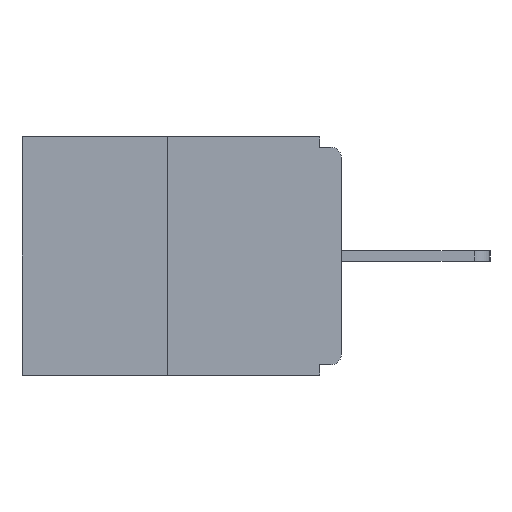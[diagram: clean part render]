
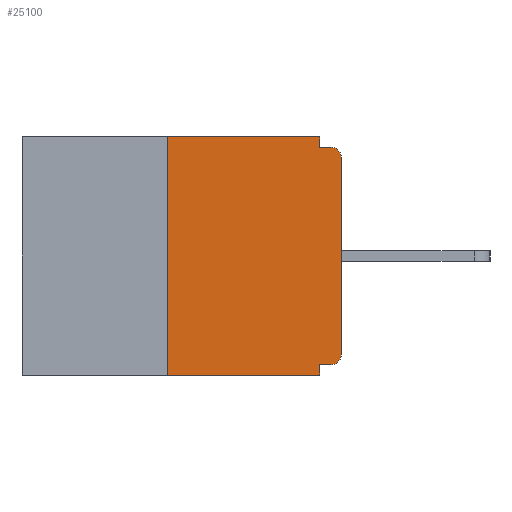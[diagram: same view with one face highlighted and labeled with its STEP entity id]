
A CAD part, left-side view. The second image highlights one B-rep face of the part: STEP entity #25100.
In plain terms, the highlighted planar face has unit normal (-1, 0, 0).
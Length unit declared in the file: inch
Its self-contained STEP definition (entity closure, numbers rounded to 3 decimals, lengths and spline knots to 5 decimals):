
#751 = CARTESIAN_POINT ( 'NONE',  ( 0., 0.031, -0.343 ) ) ;
#800 = CARTESIAN_POINT ( 'NONE',  ( 0., 0.015, -0.015 ) ) ;
#1112 = CARTESIAN_POINT ( 'NONE',  ( 0., 0.031, -0.343 ) ) ;
#2116 = CARTESIAN_POINT ( 'NONE',  ( 0., 0.46, 0. ) ) ;
#2279 = ORIENTED_EDGE ( 'NONE', *, *, #24084, .F. ) ;
#2856 = CARTESIAN_POINT ( 'NONE',  ( 0., 0.031, 0. ) ) ;
#2890 = CARTESIAN_POINT ( 'NONE',  ( 0., 0.46, -0.343 ) ) ;
#3170 = VERTEX_POINT ( 'NONE', #10653 ) ;
#3238 = CARTESIAN_POINT ( 'NONE',  ( 0., 0., -0.015 ) ) ;
#3873 = DIRECTION ( 'NONE',  ( -1., 0., 0. ) ) ;
#4693 = DIRECTION ( 'NONE',  ( 0., 1., 0. ) ) ;
#5144 = ORIENTED_EDGE ( 'NONE', *, *, #21218, .T. ) ;
#5526 = DIRECTION ( 'NONE',  ( 0., 0., -1. ) ) ;
#5822 = FACE_OUTER_BOUND ( 'NONE', #12431, .T. ) ;
#5915 = AXIS2_PLACEMENT_3D ( 'NONE', #10256, #3873, #23858 ) ;
#6657 = VECTOR ( 'NONE', #19695, 39.37008 ) ;
#6660 = VERTEX_POINT ( 'NONE', #1112 ) ;
#7017 = ORIENTED_EDGE ( 'NONE', *, *, #27545, .F. ) ;
#7025 = CARTESIAN_POINT ( 'NONE',  ( 0., 0., 0. ) ) ;
#7485 = ORIENTED_EDGE ( 'NONE', *, *, #18463, .F. ) ;
#7581 = ORIENTED_EDGE ( 'NONE', *, *, #9548, .T. ) ;
#8259 = CARTESIAN_POINT ( 'NONE',  ( 0., 0.031, -0.015 ) ) ;
#8483 = VERTEX_POINT ( 'NONE', #2856 ) ;
#8531 = ORIENTED_EDGE ( 'NONE', *, *, #17093, .F. ) ;
#8658 = VERTEX_POINT ( 'NONE', #8259 ) ;
#9449 = DIRECTION ( 'NONE',  ( 0., 0., -1. ) ) ;
#9548 = EDGE_CURVE ( 'NONE', #11157, #18806, #20333, .T. ) ;
#9725 = ORIENTED_EDGE ( 'NONE', *, *, #24787, .F. ) ;
#10256 = CARTESIAN_POINT ( 'NONE',  ( 0., 0.015, -0.03 ) ) ;
#10627 = ORIENTED_EDGE ( 'NONE', *, *, #12058, .T. ) ;
#10653 = CARTESIAN_POINT ( 'NONE',  ( 0., 0.25, 0. ) ) ;
#11157 = VERTEX_POINT ( 'NONE', #23920 ) ;
#11443 = LINE ( 'NONE', #751, #12256 ) ;
#11510 = LINE ( 'NONE', #22135, #15930 ) ;
#11767 = LINE ( 'NONE', #3238, #18440 ) ;
#11871 = DIRECTION ( 'NONE',  ( 0., -1., 0. ) ) ;
#12026 = CIRCLE ( 'NONE', #28046, 0.015 ) ;
#12058 = EDGE_CURVE ( 'NONE', #18806, #26240, #19612, .T. ) ;
#12256 = VECTOR ( 'NONE', #9449, 39.37008 ) ;
#12369 = LINE ( 'NONE', #17211, #18590 ) ;
#12431 = EDGE_LOOP ( 'NONE', ( #7485, #15846, #5144, #2279, #9725, #19965, #7581, #10627, #7017, #8531 ) ) ;
#12517 = VECTOR ( 'NONE', #11871, 39.37008 ) ;
#12832 = DIRECTION ( 'NONE',  ( 0., 0., -1. ) ) ;
#13243 = EDGE_CURVE ( 'NONE', #20688, #11157, #12026, .T. ) ;
#13969 = VECTOR ( 'NONE', #5526, 39.37008 ) ;
#14425 = CARTESIAN_POINT ( 'NONE',  ( 0., 0.031, -0.328 ) ) ;
#15404 = VERTEX_POINT ( 'NONE', #16280 ) ;
#15846 = ORIENTED_EDGE ( 'NONE', *, *, #16795, .F. ) ;
#15930 = VECTOR ( 'NONE', #4693, 39.37008 ) ;
#16280 = CARTESIAN_POINT ( 'NONE',  ( 0., 0.25, -0.343 ) ) ;
#16502 = LINE ( 'NONE', #16644, #13969 ) ;
#16644 = CARTESIAN_POINT ( 'NONE',  ( 0., 0.031, 0. ) ) ;
#16795 = EDGE_CURVE ( 'NONE', #15404, #3170, #28007, .T. ) ;
#17093 = EDGE_CURVE ( 'NONE', #8483, #8658, #16502, .T. ) ;
#17211 = CARTESIAN_POINT ( 'NONE',  ( 0., 0.46, 0. ) ) ;
#17259 = CARTESIAN_POINT ( 'NONE',  ( 0., 0.25, 0. ) ) ;
#17913 = DIRECTION ( 'NONE',  ( 0., 0., 1. ) ) ;
#18023 = CARTESIAN_POINT ( 'NONE',  ( 0., 0.015, -0.313 ) ) ;
#18440 = VECTOR ( 'NONE', #27393, 39.37008 ) ;
#18457 = LINE ( 'NONE', #2890, #12517 ) ;
#18463 = EDGE_CURVE ( 'NONE', #3170, #8483, #12369, .T. ) ;
#18590 = VECTOR ( 'NONE', #23383, 39.37008 ) ;
#18806 = VERTEX_POINT ( 'NONE', #23319 ) ;
#19026 = DIRECTION ( 'NONE',  ( 0., 0., -1. ) ) ;
#19612 = CIRCLE ( 'NONE', #5915, 0.015 ) ;
#19695 = DIRECTION ( 'NONE',  ( 0., 0., 1. ) ) ;
#19965 = ORIENTED_EDGE ( 'NONE', *, *, #13243, .T. ) ;
#20073 = AXIS2_PLACEMENT_3D ( 'NONE', #2116, #28133, #12832 ) ;
#20333 = LINE ( 'NONE', #7025, #25342 ) ;
#20688 = VERTEX_POINT ( 'NONE', #23229 ) ;
#21218 = EDGE_CURVE ( 'NONE', #15404, #6660, #18457, .T. ) ;
#21261 = PLANE ( 'NONE',  #20073 ) ;
#21760 = VERTEX_POINT ( 'NONE', #14425 ) ;
#22135 = CARTESIAN_POINT ( 'NONE',  ( 0., 0., -0.328 ) ) ;
#23229 = CARTESIAN_POINT ( 'NONE',  ( 0., 0.015, -0.328 ) ) ;
#23319 = CARTESIAN_POINT ( 'NONE',  ( 0., 0., -0.03 ) ) ;
#23383 = DIRECTION ( 'NONE',  ( 0., -1., 0. ) ) ;
#23858 = DIRECTION ( 'NONE',  ( 0., 0., -1. ) ) ;
#23920 = CARTESIAN_POINT ( 'NONE',  ( 0., 0., -0.313 ) ) ;
#24084 = EDGE_CURVE ( 'NONE', #21760, #6660, #11443, .T. ) ;
#24787 = EDGE_CURVE ( 'NONE', #20688, #21760, #11510, .T. ) ;
#25100 = ADVANCED_FACE ( 'NONE', ( #5822 ), #21261, .F. ) ;
#25342 = VECTOR ( 'NONE', #17913, 39.37008 ) ;
#26240 = VERTEX_POINT ( 'NONE', #800 ) ;
#26755 = DIRECTION ( 'NONE',  ( -1., 0., 0. ) ) ;
#27393 = DIRECTION ( 'NONE',  ( 0., -1., 0. ) ) ;
#27545 = EDGE_CURVE ( 'NONE', #8658, #26240, #11767, .T. ) ;
#28007 = LINE ( 'NONE', #17259, #6657 ) ;
#28046 = AXIS2_PLACEMENT_3D ( 'NONE', #18023, #26755, #19026 ) ;
#28133 = DIRECTION ( 'NONE',  ( 1., 0., 0. ) ) ;
